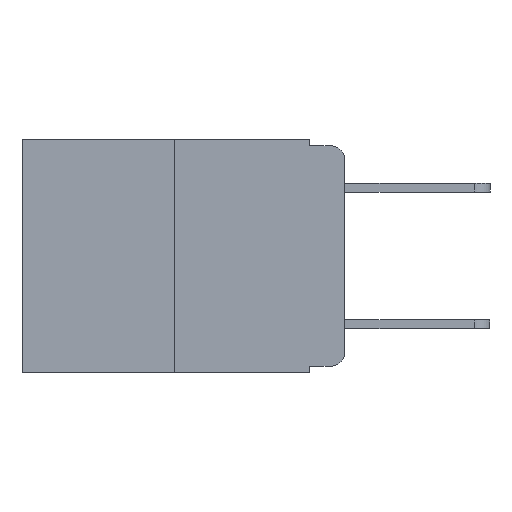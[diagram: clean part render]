
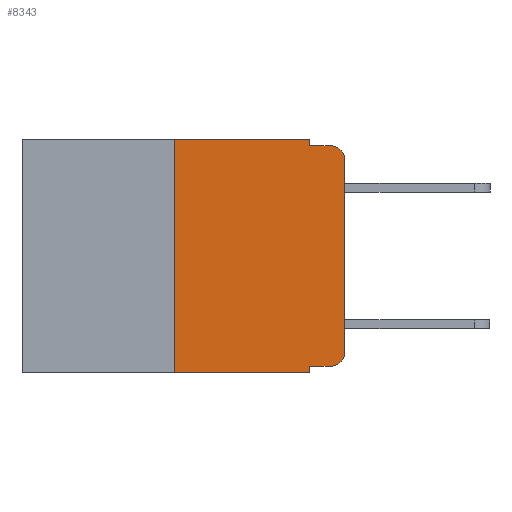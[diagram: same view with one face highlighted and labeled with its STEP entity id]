
A CAD part, left-side view. The second image highlights one B-rep face of the part: STEP entity #8343.
In plain terms, the highlighted planar face has unit normal (-1, 0, 0).
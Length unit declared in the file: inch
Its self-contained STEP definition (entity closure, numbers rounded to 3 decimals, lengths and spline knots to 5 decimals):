
#64 = ORIENTED_EDGE ( 'NONE', *, *, #4475, .F. ) ;
#231 = VECTOR ( 'NONE', #19694, 39.37008 ) ;
#237 = ORIENTED_EDGE ( 'NONE', *, *, #5286, .T. ) ;
#502 = CARTESIAN_POINT ( 'NONE',  ( 0., 0.051, -0.333 ) ) ;
#629 = CARTESIAN_POINT ( 'NONE',  ( 0., 0.02, -0.01 ) ) ;
#784 = ORIENTED_EDGE ( 'NONE', *, *, #13680, .T. ) ;
#1512 = DIRECTION ( 'NONE',  ( 0., -1., 0. ) ) ;
#1767 = VECTOR ( 'NONE', #1512, 39.37008 ) ;
#1769 = CARTESIAN_POINT ( 'NONE',  ( 0., 0.051, -0.333 ) ) ;
#2187 = EDGE_LOOP ( 'NONE', ( #784, #23600, #4108, #6729, #18384, #64, #18851, #9051, #237, #14989 ) ) ;
#2654 = VERTEX_POINT ( 'NONE', #6933 ) ;
#3075 = CARTESIAN_POINT ( 'NONE',  ( 0., 0.051, 0. ) ) ;
#3895 = LINE ( 'NONE', #15610, #22841 ) ;
#3969 = VECTOR ( 'NONE', #4386, 39.37008 ) ;
#3983 = CARTESIAN_POINT ( 'NONE',  ( 0., 0.051, 0. ) ) ;
#4108 = ORIENTED_EDGE ( 'NONE', *, *, #6572, .F. ) ;
#4163 = LINE ( 'NONE', #6281, #13491 ) ;
#4386 = DIRECTION ( 'NONE',  ( 0., -1., 0. ) ) ;
#4475 = EDGE_CURVE ( 'NONE', #17083, #13855, #11598, .T. ) ;
#4583 = AXIS2_PLACEMENT_3D ( 'NONE', #23309, #16242, #5057 ) ;
#4629 = CARTESIAN_POINT ( 'NONE',  ( 0., 0.473, -0.343 ) ) ;
#4906 = CARTESIAN_POINT ( 'NONE',  ( 0., 0., 0. ) ) ;
#5057 = DIRECTION ( 'NONE',  ( 0., 0., -1. ) ) ;
#5286 = EDGE_CURVE ( 'NONE', #6695, #14577, #10702, .T. ) ;
#5840 = DIRECTION ( 'NONE',  ( -1., 0., 0. ) ) ;
#5918 = CARTESIAN_POINT ( 'NONE',  ( 0., 0.02, -0.333 ) ) ;
#6281 = CARTESIAN_POINT ( 'NONE',  ( 0., 0.051, 0. ) ) ;
#6332 = CARTESIAN_POINT ( 'NONE',  ( 0., 0.25, 0. ) ) ;
#6517 = AXIS2_PLACEMENT_3D ( 'NONE', #17015, #5840, #18810 ) ;
#6572 = EDGE_CURVE ( 'NONE', #16673, #7572, #16731, .T. ) ;
#6664 = VERTEX_POINT ( 'NONE', #20284 ) ;
#6695 = VERTEX_POINT ( 'NONE', #1769 ) ;
#6729 = ORIENTED_EDGE ( 'NONE', *, *, #11123, .F. ) ;
#6933 = CARTESIAN_POINT ( 'NONE',  ( 0., 0.051, -0.343 ) ) ;
#7572 = VERTEX_POINT ( 'NONE', #629 ) ;
#8136 = EDGE_CURVE ( 'NONE', #6695, #2654, #4163, .T. ) ;
#8202 = DIRECTION ( 'NONE',  ( 0., -1., 0. ) ) ;
#8343 = ADVANCED_FACE ( 'NONE', ( #23362 ), #8756, .F. ) ;
#8592 = VERTEX_POINT ( 'NONE', #18738 ) ;
#8756 = PLANE ( 'NONE',  #4583 ) ;
#9051 = ORIENTED_EDGE ( 'NONE', *, *, #8136, .F. ) ;
#9192 = CIRCLE ( 'NONE', #14341, 0.02 ) ;
#9789 = EDGE_CURVE ( 'NONE', #17083, #2654, #20516, .T. ) ;
#9970 = DIRECTION ( 'NONE',  ( 0., 0., -1. ) ) ;
#10116 = DIRECTION ( 'NONE',  ( -1., 0., 0. ) ) ;
#10702 = LINE ( 'NONE', #502, #3969 ) ;
#11123 = EDGE_CURVE ( 'NONE', #22256, #16673, #11891, .T. ) ;
#11141 = CARTESIAN_POINT ( 'NONE',  ( 0., 0.25, -0.343 ) ) ;
#11598 = LINE ( 'NONE', #6332, #15988 ) ;
#11891 = LINE ( 'NONE', #3075, #21014 ) ;
#12136 = DIRECTION ( 'NONE',  ( 0., -1., 0. ) ) ;
#13264 = CARTESIAN_POINT ( 'NONE',  ( 0., 0.051, -0.01 ) ) ;
#13491 = VECTOR ( 'NONE', #9970, 39.37008 ) ;
#13518 = EDGE_CURVE ( 'NONE', #13855, #22256, #3895, .T. ) ;
#13680 = EDGE_CURVE ( 'NONE', #6664, #8592, #20068, .T. ) ;
#13855 = VERTEX_POINT ( 'NONE', #16569 ) ;
#14341 = AXIS2_PLACEMENT_3D ( 'NONE', #21052, #10116, #22832 ) ;
#14577 = VERTEX_POINT ( 'NONE', #5918 ) ;
#14989 = ORIENTED_EDGE ( 'NONE', *, *, #22877, .T. ) ;
#15610 = CARTESIAN_POINT ( 'NONE',  ( 0., 0.473, 0. ) ) ;
#15756 = VECTOR ( 'NONE', #12136, 39.37008 ) ;
#15988 = VECTOR ( 'NONE', #17479, 39.37008 ) ;
#16242 = DIRECTION ( 'NONE',  ( 1., 0., 0. ) ) ;
#16569 = CARTESIAN_POINT ( 'NONE',  ( 0., 0.25, 0. ) ) ;
#16673 = VERTEX_POINT ( 'NONE', #13264 ) ;
#16731 = LINE ( 'NONE', #23611, #1767 ) ;
#17015 = CARTESIAN_POINT ( 'NONE',  ( 0., 0.02, -0.03 ) ) ;
#17083 = VERTEX_POINT ( 'NONE', #11141 ) ;
#17479 = DIRECTION ( 'NONE',  ( 0., 0., 1. ) ) ;
#17970 = DIRECTION ( 'NONE',  ( 0., 0., -1. ) ) ;
#18384 = ORIENTED_EDGE ( 'NONE', *, *, #13518, .F. ) ;
#18738 = CARTESIAN_POINT ( 'NONE',  ( 0., 0., -0.03 ) ) ;
#18810 = DIRECTION ( 'NONE',  ( 0., 0., -1. ) ) ;
#18851 = ORIENTED_EDGE ( 'NONE', *, *, #9789, .T. ) ;
#19694 = DIRECTION ( 'NONE',  ( 0., 0., 1. ) ) ;
#19890 = CIRCLE ( 'NONE', #6517, 0.02 ) ;
#20068 = LINE ( 'NONE', #4906, #231 ) ;
#20284 = CARTESIAN_POINT ( 'NONE',  ( 0., 0., -0.313 ) ) ;
#20516 = LINE ( 'NONE', #4629, #15756 ) ;
#21014 = VECTOR ( 'NONE', #17970, 39.37008 ) ;
#21052 = CARTESIAN_POINT ( 'NONE',  ( 0., 0.02, -0.313 ) ) ;
#22227 = EDGE_CURVE ( 'NONE', #8592, #7572, #19890, .T. ) ;
#22256 = VERTEX_POINT ( 'NONE', #3983 ) ;
#22832 = DIRECTION ( 'NONE',  ( 0., 0., -1. ) ) ;
#22841 = VECTOR ( 'NONE', #8202, 39.37008 ) ;
#22877 = EDGE_CURVE ( 'NONE', #14577, #6664, #9192, .T. ) ;
#23309 = CARTESIAN_POINT ( 'NONE',  ( 0., 0.473, 0. ) ) ;
#23362 = FACE_OUTER_BOUND ( 'NONE', #2187, .T. ) ;
#23600 = ORIENTED_EDGE ( 'NONE', *, *, #22227, .T. ) ;
#23611 = CARTESIAN_POINT ( 'NONE',  ( 0., 0.051, -0.01 ) ) ;
